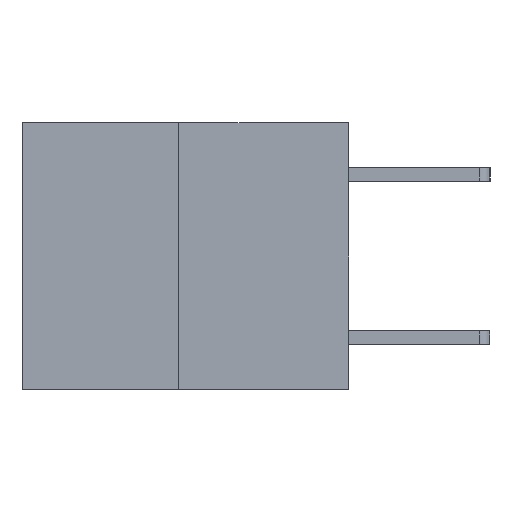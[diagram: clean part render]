
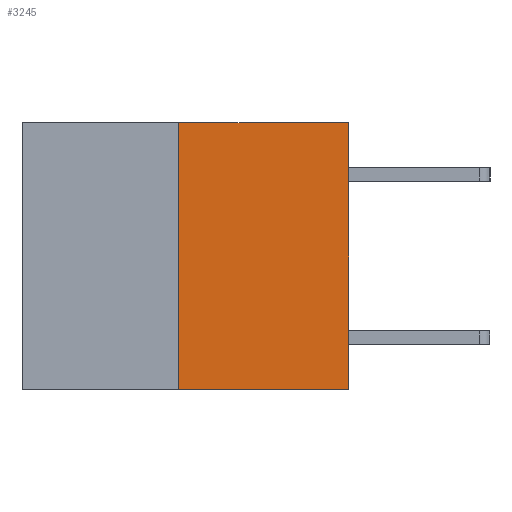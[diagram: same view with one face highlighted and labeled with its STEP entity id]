
A CAD part, left-side view. The second image highlights one B-rep face of the part: STEP entity #3245.
In plain terms, the highlighted planar face has unit normal (-1, 0, 0).
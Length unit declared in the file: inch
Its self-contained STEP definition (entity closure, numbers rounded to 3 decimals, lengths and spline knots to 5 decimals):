
#603 = ORIENTED_EDGE ( 'NONE', *, *, #1828, .T. ) ;
#992 = DIRECTION ( 'NONE',  ( 0., 0., 1. ) ) ;
#1073 = CARTESIAN_POINT ( 'NONE',  ( 0., 0.6, 0. ) ) ;
#1578 = CARTESIAN_POINT ( 'NONE',  ( 0., 0.312, 0. ) ) ;
#1828 = EDGE_CURVE ( 'NONE', #7960, #9522, #10718, .T. ) ;
#1967 = CARTESIAN_POINT ( 'NONE',  ( 0., 0.312, -0.49 ) ) ;
#2028 = VECTOR ( 'NONE', #6458, 39.37008 ) ;
#2069 = VERTEX_POINT ( 'NONE', #1578 ) ;
#2644 = VECTOR ( 'NONE', #992, 39.37008 ) ;
#2806 = DIRECTION ( 'NONE',  ( 0., -1., 0. ) ) ;
#3245 = ADVANCED_FACE ( 'NONE', ( #4803 ), #9388, .F. ) ;
#3249 = DIRECTION ( 'NONE',  ( 1., 0., 0. ) ) ;
#3522 = CARTESIAN_POINT ( 'NONE',  ( 0., 0., 0. ) ) ;
#3598 = VERTEX_POINT ( 'NONE', #10251 ) ;
#4013 = VECTOR ( 'NONE', #2806, 39.37008 ) ;
#4181 = CARTESIAN_POINT ( 'NONE',  ( 0., 0.6, 0. ) ) ;
#4803 = FACE_OUTER_BOUND ( 'NONE', #8899, .T. ) ;
#5383 = LINE ( 'NONE', #3522, #2644 ) ;
#6458 = DIRECTION ( 'NONE',  ( 0., -1., 0. ) ) ;
#6635 = ORIENTED_EDGE ( 'NONE', *, *, #7219, .F. ) ;
#6773 = DIRECTION ( 'NONE',  ( 0., 0., -1. ) ) ;
#7219 = EDGE_CURVE ( 'NONE', #2069, #3598, #11192, .T. ) ;
#7233 = EDGE_CURVE ( 'NONE', #9522, #3598, #5383, .T. ) ;
#7322 = CARTESIAN_POINT ( 'NONE',  ( 0., 0., -0.49 ) ) ;
#7329 = EDGE_CURVE ( 'NONE', #7960, #2069, #9991, .T. ) ;
#7960 = VERTEX_POINT ( 'NONE', #10959 ) ;
#8238 = ORIENTED_EDGE ( 'NONE', *, *, #7329, .F. ) ;
#8662 = VECTOR ( 'NONE', #10733, 39.37008 ) ;
#8899 = EDGE_LOOP ( 'NONE', ( #8238, #603, #8926, #6635 ) ) ;
#8926 = ORIENTED_EDGE ( 'NONE', *, *, #7233, .T. ) ;
#9388 = PLANE ( 'NONE',  #10261 ) ;
#9522 = VERTEX_POINT ( 'NONE', #7322 ) ;
#9991 = LINE ( 'NONE', #1967, #8662 ) ;
#10251 = CARTESIAN_POINT ( 'NONE',  ( 0., 0., 0. ) ) ;
#10261 = AXIS2_PLACEMENT_3D ( 'NONE', #4181, #3249, #6773 ) ;
#10718 = LINE ( 'NONE', #10728, #2028 ) ;
#10728 = CARTESIAN_POINT ( 'NONE',  ( 0., 0.6, -0.49 ) ) ;
#10733 = DIRECTION ( 'NONE',  ( 0., 0., 1. ) ) ;
#10959 = CARTESIAN_POINT ( 'NONE',  ( 0., 0.312, -0.49 ) ) ;
#11192 = LINE ( 'NONE', #1073, #4013 ) ;
